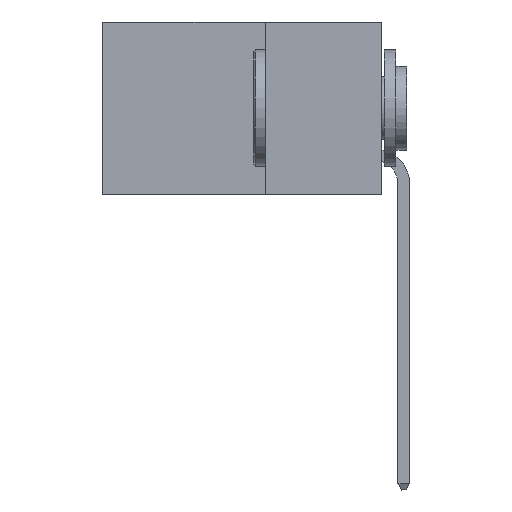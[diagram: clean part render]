
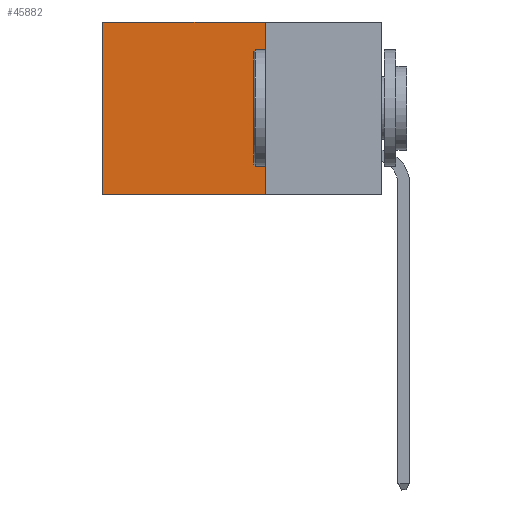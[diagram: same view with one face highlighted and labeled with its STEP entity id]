
A CAD part, left-side view. The second image highlights one B-rep face of the part: STEP entity #45882.
In plain terms, the highlighted planar face has unit normal (-1, 0, 0).
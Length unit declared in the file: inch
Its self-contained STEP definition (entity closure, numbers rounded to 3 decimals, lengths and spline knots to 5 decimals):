
#2899 = AXIS2_PLACEMENT_3D ( 'NONE', #15806, #40161, #22779 ) ;
#5414 = CARTESIAN_POINT ( 'NONE',  ( 0.2875, 0.6, -0.37 ) ) ;
#8596 = FACE_OUTER_BOUND ( 'NONE', #26885, .T. ) ;
#10171 = DIRECTION ( 'NONE',  ( 0., 0., -1. ) ) ;
#10985 = VECTOR ( 'NONE', #10171, 39.37008 ) ;
#11871 = VECTOR ( 'NONE', #22269, 39.37008 ) ;
#12224 = VERTEX_POINT ( 'NONE', #5414 ) ;
#13607 = VECTOR ( 'NONE', #38287, 39.37008 ) ;
#14407 = VECTOR ( 'NONE', #38514, 39.37008 ) ;
#14612 = LINE ( 'NONE', #27081, #11871 ) ;
#15242 = EDGE_CURVE ( 'NONE', #32907, #43834, #27619, .T. ) ;
#15604 = CARTESIAN_POINT ( 'NONE',  ( 0.2875, 0.25, -0.37 ) ) ;
#15806 = CARTESIAN_POINT ( 'NONE',  ( 0.2875, 0.25, 0. ) ) ;
#17155 = CARTESIAN_POINT ( 'NONE',  ( 0.2875, 0.25, 0. ) ) ;
#20192 = VERTEX_POINT ( 'NONE', #30032 ) ;
#21173 = CARTESIAN_POINT ( 'NONE',  ( 0.2875, 0.25, 0. ) ) ;
#22199 = ORIENTED_EDGE ( 'NONE', *, *, #23282, .T. ) ;
#22269 = DIRECTION ( 'NONE',  ( 0., 0., -1. ) ) ;
#22779 = DIRECTION ( 'NONE',  ( 0., 0., -1. ) ) ;
#23282 = EDGE_CURVE ( 'NONE', #20192, #12224, #14612, .T. ) ;
#24158 = LINE ( 'NONE', #24192, #13607 ) ;
#24192 = CARTESIAN_POINT ( 'NONE',  ( 0.2875, 0.25, -0.37 ) ) ;
#24418 = LINE ( 'NONE', #17155, #14407 ) ;
#26885 = EDGE_LOOP ( 'NONE', ( #22199, #42587, #44559, #30841 ) ) ;
#27081 = CARTESIAN_POINT ( 'NONE',  ( 0.2875, 0.6, 0. ) ) ;
#27619 = LINE ( 'NONE', #21173, #10985 ) ;
#29863 = EDGE_CURVE ( 'NONE', #32907, #20192, #24418, .T. ) ;
#30032 = CARTESIAN_POINT ( 'NONE',  ( 0.2875, 0.6, 0. ) ) ;
#30841 = ORIENTED_EDGE ( 'NONE', *, *, #29863, .T. ) ;
#32907 = VERTEX_POINT ( 'NONE', #45912 ) ;
#38287 = DIRECTION ( 'NONE',  ( 0., 1., 0. ) ) ;
#38514 = DIRECTION ( 'NONE',  ( 0., 1., 0. ) ) ;
#40161 = DIRECTION ( 'NONE',  ( 1., 0., 0. ) ) ;
#40309 = PLANE ( 'NONE',  #2899 ) ;
#42587 = ORIENTED_EDGE ( 'NONE', *, *, #45499, .F. ) ;
#43834 = VERTEX_POINT ( 'NONE', #15604 ) ;
#44559 = ORIENTED_EDGE ( 'NONE', *, *, #15242, .F. ) ;
#45499 = EDGE_CURVE ( 'NONE', #43834, #12224, #24158, .T. ) ;
#45882 = ADVANCED_FACE ( 'NONE', ( #8596 ), #40309, .F. ) ;
#45912 = CARTESIAN_POINT ( 'NONE',  ( 0.2875, 0.25, 0. ) ) ;
